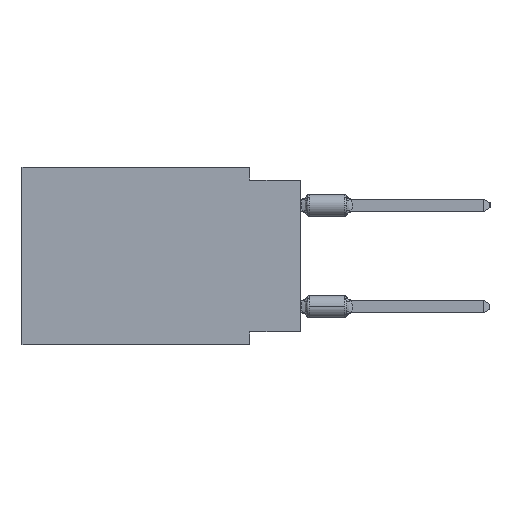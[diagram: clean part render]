
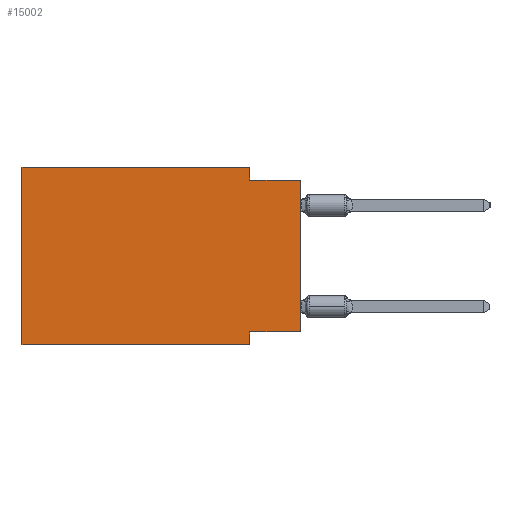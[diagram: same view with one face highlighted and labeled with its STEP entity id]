
A CAD part, left-side view. The second image highlights one B-rep face of the part: STEP entity #15002.
In plain terms, the highlighted planar face has unit normal (-1, 0, 0).
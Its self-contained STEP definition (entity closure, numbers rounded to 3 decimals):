
#450 = EDGE_CURVE ( 'NONE', #25893, #25177, #36690, .T. ) ;
#846 = CARTESIAN_POINT ( 'NONE',  ( 0., 13.97, 0. ) ) ;
#2672 = VECTOR ( 'NONE', #8580, 1000. ) ;
#3101 = VECTOR ( 'NONE', #35448, 1000. ) ;
#4363 = EDGE_CURVE ( 'NONE', #17440, #10755, #15296, .T. ) ;
#4637 = DIRECTION ( 'NONE',  ( 0., 0., -1. ) ) ;
#4783 = PLANE ( 'NONE',  #6942 ) ;
#5266 = LINE ( 'NONE', #25908, #33193 ) ;
#5751 = VECTOR ( 'NONE', #15892, 1000. ) ;
#6583 = LINE ( 'NONE', #9916, #19942 ) ;
#6838 = CARTESIAN_POINT ( 'NONE',  ( 0., 2.54, 0. ) ) ;
#6942 = AXIS2_PLACEMENT_3D ( 'NONE', #25991, #22665, #14009 ) ;
#6989 = ORIENTED_EDGE ( 'NONE', *, *, #450, .F. ) ;
#7344 = EDGE_CURVE ( 'NONE', #38772, #19595, #24280, .T. ) ;
#8580 = DIRECTION ( 'NONE',  ( 0., 0., 1. ) ) ;
#9209 = CARTESIAN_POINT ( 'NONE',  ( 0., 13.97, -8.89 ) ) ;
#9539 = DIRECTION ( 'NONE',  ( 0., -1., 0. ) ) ;
#9562 = CARTESIAN_POINT ( 'NONE',  ( 0., 13.97, 0. ) ) ;
#9916 = CARTESIAN_POINT ( 'NONE',  ( 0., 13.97, 0. ) ) ;
#10755 = VERTEX_POINT ( 'NONE', #13150 ) ;
#12561 = VECTOR ( 'NONE', #33486, 1000. ) ;
#13150 = CARTESIAN_POINT ( 'NONE',  ( 0., 2.54, -0.635 ) ) ;
#14009 = DIRECTION ( 'NONE',  ( 0., 0., -1. ) ) ;
#14209 = CARTESIAN_POINT ( 'NONE',  ( 0., 0., -0.635 ) ) ;
#14580 = EDGE_CURVE ( 'NONE', #35934, #24392, #31580, .T. ) ;
#15002 = ADVANCED_FACE ( 'NONE', ( #16960 ), #4783, .F. ) ;
#15296 = LINE ( 'NONE', #6838, #5751 ) ;
#15853 = DIRECTION ( 'NONE',  ( 0., 0., 1. ) ) ;
#15892 = DIRECTION ( 'NONE',  ( 0., 0., -1. ) ) ;
#16575 = VECTOR ( 'NONE', #15853, 1000. ) ;
#16960 = FACE_OUTER_BOUND ( 'NONE', #17970, .T. ) ;
#17011 = CARTESIAN_POINT ( 'NONE',  ( 0., 2.54, -8.89 ) ) ;
#17165 = LINE ( 'NONE', #14209, #3101 ) ;
#17254 = DIRECTION ( 'NONE',  ( 0., -1., 0. ) ) ;
#17440 = VERTEX_POINT ( 'NONE', #36936 ) ;
#17970 = EDGE_LOOP ( 'NONE', ( #23914, #22318, #29957, #26149, #6989, #36369, #33108, #30752 ) ) ;
#18393 = CARTESIAN_POINT ( 'NONE',  ( 0., 0., -0.635 ) ) ;
#19320 = CARTESIAN_POINT ( 'NONE',  ( 0., 0., -8.255 ) ) ;
#19595 = VERTEX_POINT ( 'NONE', #18393 ) ;
#19624 = EDGE_CURVE ( 'NONE', #25177, #17440, #6583, .T. ) ;
#19722 = CARTESIAN_POINT ( 'NONE',  ( 0., 2.54, -8.255 ) ) ;
#19942 = VECTOR ( 'NONE', #9539, 1000. ) ;
#20963 = CARTESIAN_POINT ( 'NONE',  ( 0., 0., 0. ) ) ;
#22214 = CARTESIAN_POINT ( 'NONE',  ( 0., 2.54, -8.89 ) ) ;
#22318 = ORIENTED_EDGE ( 'NONE', *, *, #38362, .F. ) ;
#22665 = DIRECTION ( 'NONE',  ( 1., 0., 0. ) ) ;
#23012 = CARTESIAN_POINT ( 'NONE',  ( 0., 0., -8.255 ) ) ;
#23914 = ORIENTED_EDGE ( 'NONE', *, *, #7344, .T. ) ;
#24005 = EDGE_CURVE ( 'NONE', #38772, #35934, #30527, .T. ) ;
#24280 = LINE ( 'NONE', #20963, #2672 ) ;
#24392 = VERTEX_POINT ( 'NONE', #22214 ) ;
#25177 = VERTEX_POINT ( 'NONE', #846 ) ;
#25893 = VERTEX_POINT ( 'NONE', #9209 ) ;
#25908 = CARTESIAN_POINT ( 'NONE',  ( 0., 13.97, -8.89 ) ) ;
#25991 = CARTESIAN_POINT ( 'NONE',  ( 0., 13.97, 0. ) ) ;
#26149 = ORIENTED_EDGE ( 'NONE', *, *, #19624, .F. ) ;
#28412 = EDGE_CURVE ( 'NONE', #25893, #24392, #5266, .T. ) ;
#29957 = ORIENTED_EDGE ( 'NONE', *, *, #4363, .F. ) ;
#30527 = LINE ( 'NONE', #19320, #12561 ) ;
#30750 = VECTOR ( 'NONE', #4637, 1000. ) ;
#30752 = ORIENTED_EDGE ( 'NONE', *, *, #24005, .F. ) ;
#31580 = LINE ( 'NONE', #17011, #30750 ) ;
#33108 = ORIENTED_EDGE ( 'NONE', *, *, #14580, .F. ) ;
#33193 = VECTOR ( 'NONE', #17254, 1000. ) ;
#33486 = DIRECTION ( 'NONE',  ( 0., 1., 0. ) ) ;
#35448 = DIRECTION ( 'NONE',  ( 0., -1., 0. ) ) ;
#35934 = VERTEX_POINT ( 'NONE', #19722 ) ;
#36369 = ORIENTED_EDGE ( 'NONE', *, *, #28412, .T. ) ;
#36690 = LINE ( 'NONE', #9562, #16575 ) ;
#36936 = CARTESIAN_POINT ( 'NONE',  ( 0., 2.54, 0. ) ) ;
#38362 = EDGE_CURVE ( 'NONE', #10755, #19595, #17165, .T. ) ;
#38772 = VERTEX_POINT ( 'NONE', #23012 ) ;
